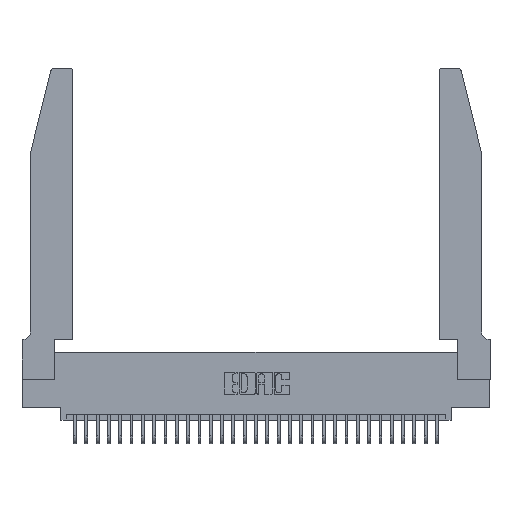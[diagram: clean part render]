
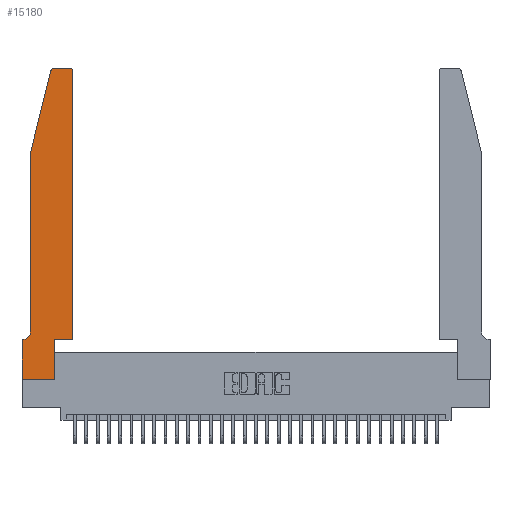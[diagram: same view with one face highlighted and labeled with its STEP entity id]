
A CAD part, top view. The second image highlights one B-rep face of the part: STEP entity #15180.
In plain terms, the highlighted planar face has unit normal (0, 0, 1).
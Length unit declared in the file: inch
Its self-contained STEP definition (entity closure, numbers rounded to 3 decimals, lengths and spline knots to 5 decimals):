
#136 = VECTOR ( 'NONE', #3938, 39.37008 ) ;
#865 = CARTESIAN_POINT ( 'NONE',  ( 0.25487, 2.72718, 0.37 ) ) ;
#1365 = VERTEX_POINT ( 'NONE', #6052 ) ;
#2858 = VECTOR ( 'NONE', #5367, 39.37008 ) ;
#3265 = EDGE_CURVE ( 'NONE', #27673, #27338, #18109, .T. ) ;
#3487 = CIRCLE ( 'NONE', #10261, 0.03 ) ;
#3938 = DIRECTION ( 'NONE',  ( 0., 1., 0. ) ) ;
#4026 = DIRECTION ( 'NONE',  ( 0., 0., -1. ) ) ;
#4172 = LINE ( 'NONE', #17259, #27373 ) ;
#5022 = ORIENTED_EDGE ( 'NONE', *, *, #17085, .T. ) ;
#5179 = ORIENTED_EDGE ( 'NONE', *, *, #18737, .T. ) ;
#5367 = DIRECTION ( 'NONE',  ( -0.239, -0.971, 0. ) ) ;
#5582 = CARTESIAN_POINT ( 'NONE',  ( 0.4205, 2.72, 0.37 ) ) ;
#5661 = CARTESIAN_POINT ( 'NONE',  ( 0.2865, 0.35, 0.37 ) ) ;
#5824 = FACE_OUTER_BOUND ( 'NONE', #24140, .T. ) ;
#5872 = ORIENTED_EDGE ( 'NONE', *, *, #8235, .T. ) ;
#5950 = CARTESIAN_POINT ( 'NONE',  ( 0.0755, 2., 0.37 ) ) ;
#6052 = CARTESIAN_POINT ( 'NONE',  ( 0.0755, 0.42, 0.37 ) ) ;
#6074 = CARTESIAN_POINT ( 'NONE',  ( 0., 0., 0.37 ) ) ;
#6261 = ORIENTED_EDGE ( 'NONE', *, *, #33294, .T. ) ;
#6555 = DIRECTION ( 'NONE',  ( -1., 0., 0. ) ) ;
#6674 = CARTESIAN_POINT ( 'NONE',  ( 0.2605, 2.75, 0.37 ) ) ;
#6727 = VERTEX_POINT ( 'NONE', #19567 ) ;
#7296 = LINE ( 'NONE', #6674, #16227 ) ;
#7472 = DIRECTION ( 'NONE',  ( -1., 0., 0. ) ) ;
#7679 = VERTEX_POINT ( 'NONE', #865 ) ;
#7918 = EDGE_CURVE ( 'NONE', #13828, #7679, #32714, .T. ) ;
#8235 = EDGE_CURVE ( 'NONE', #32637, #17017, #26558, .T. ) ;
#8789 = AXIS2_PLACEMENT_3D ( 'NONE', #19617, #4026, #17316 ) ;
#9283 = CARTESIAN_POINT ( 'NONE',  ( 0.4505, 0.35, 0.37 ) ) ;
#9704 = CARTESIAN_POINT ( 'NONE',  ( 0.284, 2.72, 0.37 ) ) ;
#10033 = DIRECTION ( 'NONE',  ( 0., 0., 1. ) ) ;
#10117 = ORIENTED_EDGE ( 'NONE', *, *, #14059, .T. ) ;
#10261 = AXIS2_PLACEMENT_3D ( 'NONE', #5582, #10966, #28719 ) ;
#10468 = EDGE_CURVE ( 'NONE', #26732, #13828, #7296, .T. ) ;
#10966 = DIRECTION ( 'NONE',  ( 0., 0., 1. ) ) ;
#11023 = LINE ( 'NONE', #29010, #18292 ) ;
#12190 = DIRECTION ( 'NONE',  ( 1., 0., 0. ) ) ;
#13125 = DIRECTION ( 'NONE',  ( 1., 0., 0. ) ) ;
#13552 = DIRECTION ( 'NONE',  ( 0., -1., 0. ) ) ;
#13733 = VERTEX_POINT ( 'NONE', #21215 ) ;
#13828 = VERTEX_POINT ( 'NONE', #26656 ) ;
#14059 = EDGE_CURVE ( 'NONE', #1365, #13733, #16448, .T. ) ;
#14379 = CARTESIAN_POINT ( 'NONE',  ( 0., 0., 0.37 ) ) ;
#15180 = ADVANCED_FACE ( 'NONE', ( #5824 ), #33178, .T. ) ;
#15301 = VECTOR ( 'NONE', #16348, 39.37008 ) ;
#15941 = EDGE_CURVE ( 'NONE', #25130, #32637, #33522, .T. ) ;
#16080 = DIRECTION ( 'NONE',  ( 0., 1., 0. ) ) ;
#16206 = EDGE_CURVE ( 'NONE', #13733, #27673, #4172, .T. ) ;
#16227 = VECTOR ( 'NONE', #6555, 39.37008 ) ;
#16348 = DIRECTION ( 'NONE',  ( 1., 0., 0. ) ) ;
#16394 = VECTOR ( 'NONE', #13125, 39.37008 ) ;
#16448 = CIRCLE ( 'NONE', #8789, 0.07 ) ;
#17017 = VERTEX_POINT ( 'NONE', #33075 ) ;
#17085 = EDGE_CURVE ( 'NONE', #7679, #30661, #18288, .T. ) ;
#17111 = ORIENTED_EDGE ( 'NONE', *, *, #7918, .T. ) ;
#17259 = CARTESIAN_POINT ( 'NONE',  ( 0.0755, 0.35, 0.37 ) ) ;
#17316 = DIRECTION ( 'NONE',  ( -1., 0., 0. ) ) ;
#17319 = VECTOR ( 'NONE', #21977, 39.37008 ) ;
#17652 = DIRECTION ( 'NONE',  ( 0., 0., 1. ) ) ;
#18109 = LINE ( 'NONE', #14379, #17319 ) ;
#18288 = LINE ( 'NONE', #22699, #2858 ) ;
#18292 = VECTOR ( 'NONE', #13552, 39.37008 ) ;
#18737 = EDGE_CURVE ( 'NONE', #30661, #1365, #11023, .T. ) ;
#18828 = AXIS2_PLACEMENT_3D ( 'NONE', #22785, #17652, #22885 ) ;
#19083 = ORIENTED_EDGE ( 'NONE', *, *, #10468, .T. ) ;
#19486 = CARTESIAN_POINT ( 'NONE',  ( 0., 0., 0.37 ) ) ;
#19567 = CARTESIAN_POINT ( 'NONE',  ( 0.2865, 0., 0.37 ) ) ;
#19617 = CARTESIAN_POINT ( 'NONE',  ( 0.0055, 0.42, 0.37 ) ) ;
#19668 = VECTOR ( 'NONE', #16080, 39.37008 ) ;
#20246 = ORIENTED_EDGE ( 'NONE', *, *, #3265, .T. ) ;
#21215 = CARTESIAN_POINT ( 'NONE',  ( 0.0055, 0.35, 0.37 ) ) ;
#21321 = EDGE_CURVE ( 'NONE', #27338, #6727, #25845, .T. ) ;
#21502 = ORIENTED_EDGE ( 'NONE', *, *, #15941, .T. ) ;
#21915 = CARTESIAN_POINT ( 'NONE',  ( 0.4205, 2.75, 0.37 ) ) ;
#21977 = DIRECTION ( 'NONE',  ( 0., -1., 0. ) ) ;
#22699 = CARTESIAN_POINT ( 'NONE',  ( 0.0755, 2., 0.37 ) ) ;
#22785 = CARTESIAN_POINT ( 'NONE',  ( 0., 0.35, 0.37 ) ) ;
#22885 = DIRECTION ( 'NONE',  ( 1., 0., 0. ) ) ;
#24064 = EDGE_CURVE ( 'NONE', #6727, #25130, #32281, .T. ) ;
#24140 = EDGE_LOOP ( 'NONE', ( #19083, #17111, #5022, #5179, #10117, #33559, #20246, #32878, #26912, #21502, #5872, #6261 ) ) ;
#25130 = VERTEX_POINT ( 'NONE', #5661 ) ;
#25845 = LINE ( 'NONE', #6074, #15301 ) ;
#25958 = AXIS2_PLACEMENT_3D ( 'NONE', #9704, #10033, #12190 ) ;
#26413 = CARTESIAN_POINT ( 'NONE',  ( 0.4505, 0.35, 0.37 ) ) ;
#26558 = LINE ( 'NONE', #26413, #19668 ) ;
#26656 = CARTESIAN_POINT ( 'NONE',  ( 0.284, 2.75, 0.37 ) ) ;
#26732 = VERTEX_POINT ( 'NONE', #21915 ) ;
#26912 = ORIENTED_EDGE ( 'NONE', *, *, #24064, .T. ) ;
#27338 = VERTEX_POINT ( 'NONE', #19486 ) ;
#27373 = VECTOR ( 'NONE', #7472, 39.37008 ) ;
#27673 = VERTEX_POINT ( 'NONE', #28126 ) ;
#28126 = CARTESIAN_POINT ( 'NONE',  ( 0., 0.35, 0.37 ) ) ;
#28719 = DIRECTION ( 'NONE',  ( 1., 0., 0. ) ) ;
#29010 = CARTESIAN_POINT ( 'NONE',  ( 0.0755, 2., 0.37 ) ) ;
#29882 = CARTESIAN_POINT ( 'NONE',  ( 0.2865, 0.35, 0.37 ) ) ;
#30661 = VERTEX_POINT ( 'NONE', #5950 ) ;
#30822 = CARTESIAN_POINT ( 'NONE',  ( 0.4505, 0.35, 0.37 ) ) ;
#32281 = LINE ( 'NONE', #29882, #136 ) ;
#32637 = VERTEX_POINT ( 'NONE', #30822 ) ;
#32714 = CIRCLE ( 'NONE', #25958, 0.03 ) ;
#32878 = ORIENTED_EDGE ( 'NONE', *, *, #21321, .T. ) ;
#33075 = CARTESIAN_POINT ( 'NONE',  ( 0.4505, 2.72, 0.37 ) ) ;
#33178 = PLANE ( 'NONE',  #18828 ) ;
#33294 = EDGE_CURVE ( 'NONE', #17017, #26732, #3487, .T. ) ;
#33522 = LINE ( 'NONE', #9283, #16394 ) ;
#33559 = ORIENTED_EDGE ( 'NONE', *, *, #16206, .T. ) ;
